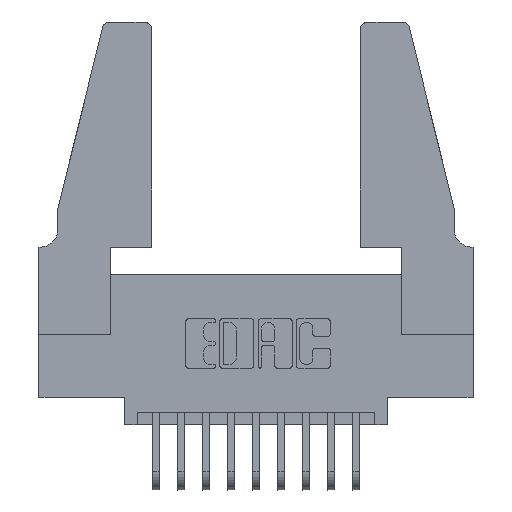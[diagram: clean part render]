
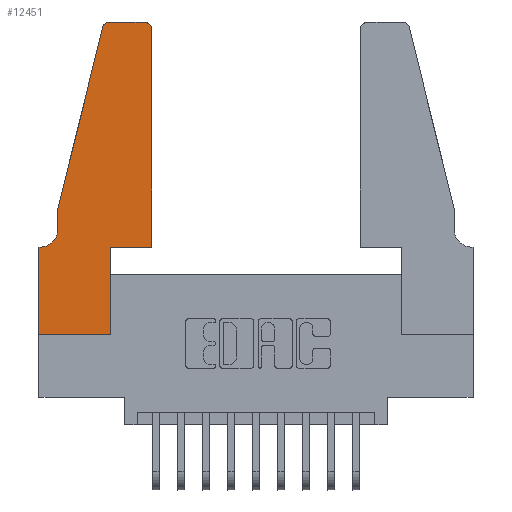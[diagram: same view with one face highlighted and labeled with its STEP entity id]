
A CAD part, top view. The second image highlights one B-rep face of the part: STEP entity #12451.
In plain terms, the highlighted planar face has unit normal (0, 0, 1).
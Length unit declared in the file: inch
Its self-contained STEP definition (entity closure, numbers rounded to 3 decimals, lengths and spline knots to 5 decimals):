
#148 = DIRECTION ( 'NONE',  ( 0., -1., 0. ) ) ;
#226 = DIRECTION ( 'NONE',  ( 1., 0., 0. ) ) ;
#390 = CARTESIAN_POINT ( 'NONE',  ( 0.2605, 1.25, 0.37 ) ) ;
#702 = CARTESIAN_POINT ( 'NONE',  ( 0.0055, 0.35, 0.37 ) ) ;
#807 = VECTOR ( 'NONE', #11688, 39.37008 ) ;
#1587 = EDGE_CURVE ( 'NONE', #13191, #13281, #5836, .T. ) ;
#1764 = CARTESIAN_POINT ( 'NONE',  ( 0.0755, 0.42, 0.37 ) ) ;
#2001 = DIRECTION ( 'NONE',  ( 1., 0., 0. ) ) ;
#2094 = VERTEX_POINT ( 'NONE', #9181 ) ;
#2095 = EDGE_CURVE ( 'NONE', #12982, #2094, #9633, .T. ) ;
#2359 = EDGE_CURVE ( 'NONE', #2094, #11352, #11448, .T. ) ;
#2577 = VECTOR ( 'NONE', #5601, 39.37008 ) ;
#2599 = CARTESIAN_POINT ( 'NONE',  ( 0.4505, 1.22, 0.37 ) ) ;
#2722 = EDGE_CURVE ( 'NONE', #13281, #5638, #9778, .T. ) ;
#2788 = DIRECTION ( 'NONE',  ( -1., 0., 0. ) ) ;
#2962 = VERTEX_POINT ( 'NONE', #8965 ) ;
#3232 = ORIENTED_EDGE ( 'NONE', *, *, #13339, .T. ) ;
#3743 = EDGE_CURVE ( 'NONE', #6629, #10877, #8627, .T. ) ;
#4002 = CARTESIAN_POINT ( 'NONE',  ( 0.4505, 0.35, 0.37 ) ) ;
#4021 = CARTESIAN_POINT ( 'NONE',  ( 0.4505, 0.35, 0.37 ) ) ;
#4106 = VECTOR ( 'NONE', #11494, 39.37008 ) ;
#4150 = CARTESIAN_POINT ( 'NONE',  ( 0.2865, 0.35, 0.37 ) ) ;
#4165 = ORIENTED_EDGE ( 'NONE', *, *, #8362, .T. ) ;
#4269 = CARTESIAN_POINT ( 'NONE',  ( 0.4205, 1.22, 0.37 ) ) ;
#4673 = CARTESIAN_POINT ( 'NONE',  ( 0.2865, 0.35, 0.37 ) ) ;
#4787 = VERTEX_POINT ( 'NONE', #7740 ) ;
#4987 = EDGE_CURVE ( 'NONE', #5638, #11376, #7058, .T. ) ;
#5594 = LINE ( 'NONE', #8473, #5764 ) ;
#5601 = DIRECTION ( 'NONE',  ( -0.239, -0.971, 0. ) ) ;
#5638 = VERTEX_POINT ( 'NONE', #702 ) ;
#5764 = VECTOR ( 'NONE', #148, 39.37008 ) ;
#5836 = LINE ( 'NONE', #15179, #13717 ) ;
#5965 = DIRECTION ( 'NONE',  ( 0., -1., 0. ) ) ;
#6264 = ORIENTED_EDGE ( 'NONE', *, *, #13510, .T. ) ;
#6399 = CARTESIAN_POINT ( 'NONE',  ( 0.0755, 0.5, 0.37 ) ) ;
#6575 = LINE ( 'NONE', #4002, #10907 ) ;
#6629 = VERTEX_POINT ( 'NONE', #12384 ) ;
#6738 = DIRECTION ( 'NONE',  ( 0., 0., 1. ) ) ;
#6867 = CARTESIAN_POINT ( 'NONE',  ( 0., 0., 0.37 ) ) ;
#6912 = ORIENTED_EDGE ( 'NONE', *, *, #11326, .T. ) ;
#6934 = VECTOR ( 'NONE', #2788, 39.37008 ) ;
#7058 = LINE ( 'NONE', #13844, #7641 ) ;
#7641 = VECTOR ( 'NONE', #8999, 39.37008 ) ;
#7714 = PLANE ( 'NONE',  #13346 ) ;
#7740 = CARTESIAN_POINT ( 'NONE',  ( 0.25487, 1.22718, 0.37 ) ) ;
#7837 = CIRCLE ( 'NONE', #14180, 0.03 ) ;
#7845 = CARTESIAN_POINT ( 'NONE',  ( 0.4505, 0.35, 0.37 ) ) ;
#7928 = CARTESIAN_POINT ( 'NONE',  ( 0., 0.35, 0.37 ) ) ;
#8076 = VECTOR ( 'NONE', #14924, 39.37008 ) ;
#8260 = AXIS2_PLACEMENT_3D ( 'NONE', #12656, #11664, #13833 ) ;
#8362 = EDGE_CURVE ( 'NONE', #4787, #13191, #14175, .T. ) ;
#8473 = CARTESIAN_POINT ( 'NONE',  ( 0., 0., 0.37 ) ) ;
#8627 = LINE ( 'NONE', #4150, #8076 ) ;
#8722 = DIRECTION ( 'NONE',  ( 0., 1., 0. ) ) ;
#8927 = ORIENTED_EDGE ( 'NONE', *, *, #2095, .T. ) ;
#8965 = CARTESIAN_POINT ( 'NONE',  ( 0., 0., 0.37 ) ) ;
#8999 = DIRECTION ( 'NONE',  ( -1., 0., 0. ) ) ;
#9181 = CARTESIAN_POINT ( 'NONE',  ( 0.4205, 1.25, 0.37 ) ) ;
#9220 = EDGE_LOOP ( 'NONE', ( #12277, #11266, #4165, #9905, #12294, #10919, #6264, #6912, #13651, #3232, #13272, #8927 ) ) ;
#9387 = LINE ( 'NONE', #7845, #4106 ) ;
#9633 = CIRCLE ( 'NONE', #9920, 0.03 ) ;
#9692 = CARTESIAN_POINT ( 'NONE',  ( 0., 0.35, 0.37 ) ) ;
#9778 = CIRCLE ( 'NONE', #8260, 0.07 ) ;
#9905 = ORIENTED_EDGE ( 'NONE', *, *, #1587, .T. ) ;
#9920 = AXIS2_PLACEMENT_3D ( 'NONE', #4269, #12625, #14057 ) ;
#10315 = CARTESIAN_POINT ( 'NONE',  ( 0.0755, 0.5, 0.37 ) ) ;
#10877 = VERTEX_POINT ( 'NONE', #4673 ) ;
#10907 = VECTOR ( 'NONE', #8722, 39.37008 ) ;
#10919 = ORIENTED_EDGE ( 'NONE', *, *, #4987, .T. ) ;
#11013 = VERTEX_POINT ( 'NONE', #4021 ) ;
#11266 = ORIENTED_EDGE ( 'NONE', *, *, #14110, .T. ) ;
#11326 = EDGE_CURVE ( 'NONE', #2962, #6629, #13347, .T. ) ;
#11352 = VERTEX_POINT ( 'NONE', #11994 ) ;
#11376 = VERTEX_POINT ( 'NONE', #9692 ) ;
#11448 = LINE ( 'NONE', #390, #6934 ) ;
#11494 = DIRECTION ( 'NONE',  ( 1., 0., 0. ) ) ;
#11664 = DIRECTION ( 'NONE',  ( 0., 0., -1. ) ) ;
#11688 = DIRECTION ( 'NONE',  ( 1., 0., 0. ) ) ;
#11994 = CARTESIAN_POINT ( 'NONE',  ( 0.284, 1.25, 0.37 ) ) ;
#12080 = DIRECTION ( 'NONE',  ( 0., 0., 1. ) ) ;
#12127 = CARTESIAN_POINT ( 'NONE',  ( 0.284, 1.22, 0.37 ) ) ;
#12223 = EDGE_CURVE ( 'NONE', #11013, #12982, #6575, .T. ) ;
#12277 = ORIENTED_EDGE ( 'NONE', *, *, #2359, .T. ) ;
#12294 = ORIENTED_EDGE ( 'NONE', *, *, #2722, .T. ) ;
#12384 = CARTESIAN_POINT ( 'NONE',  ( 0.2865, 0., 0.37 ) ) ;
#12451 = ADVANCED_FACE ( 'NONE', ( #13615 ), #7714, .T. ) ;
#12625 = DIRECTION ( 'NONE',  ( 0., 0., 1. ) ) ;
#12656 = CARTESIAN_POINT ( 'NONE',  ( 0.0055, 0.42, 0.37 ) ) ;
#12982 = VERTEX_POINT ( 'NONE', #2599 ) ;
#13191 = VERTEX_POINT ( 'NONE', #6399 ) ;
#13272 = ORIENTED_EDGE ( 'NONE', *, *, #12223, .T. ) ;
#13281 = VERTEX_POINT ( 'NONE', #1764 ) ;
#13339 = EDGE_CURVE ( 'NONE', #10877, #11013, #9387, .T. ) ;
#13346 = AXIS2_PLACEMENT_3D ( 'NONE', #7928, #6738, #2001 ) ;
#13347 = LINE ( 'NONE', #6867, #807 ) ;
#13510 = EDGE_CURVE ( 'NONE', #11376, #2962, #5594, .T. ) ;
#13615 = FACE_OUTER_BOUND ( 'NONE', #9220, .T. ) ;
#13651 = ORIENTED_EDGE ( 'NONE', *, *, #3743, .T. ) ;
#13717 = VECTOR ( 'NONE', #5965, 39.37008 ) ;
#13833 = DIRECTION ( 'NONE',  ( -1., 0., 0. ) ) ;
#13844 = CARTESIAN_POINT ( 'NONE',  ( 0.0755, 0.35, 0.37 ) ) ;
#14057 = DIRECTION ( 'NONE',  ( 1., 0., 0. ) ) ;
#14110 = EDGE_CURVE ( 'NONE', #11352, #4787, #7837, .T. ) ;
#14175 = LINE ( 'NONE', #10315, #2577 ) ;
#14180 = AXIS2_PLACEMENT_3D ( 'NONE', #12127, #12080, #226 ) ;
#14924 = DIRECTION ( 'NONE',  ( 0., 1., 0. ) ) ;
#15179 = CARTESIAN_POINT ( 'NONE',  ( 0.0755, 0.5, 0.37 ) ) ;
